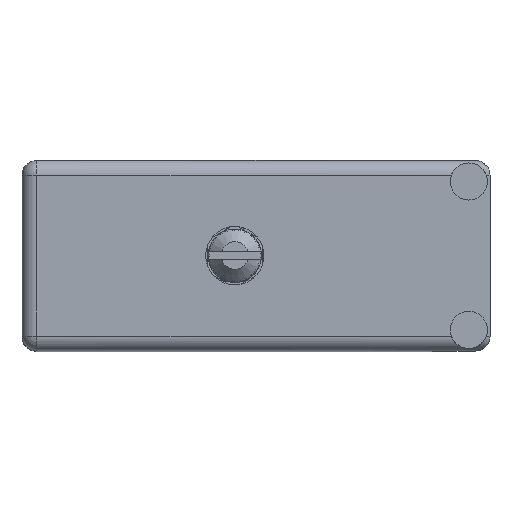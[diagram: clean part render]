
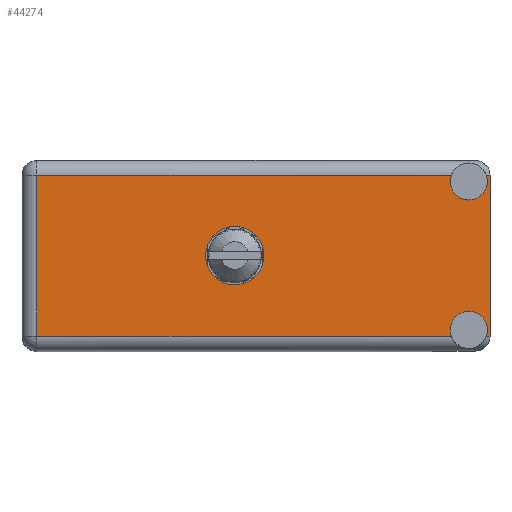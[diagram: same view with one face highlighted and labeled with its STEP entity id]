
A CAD part, top view. The second image highlights one B-rep face of the part: STEP entity #44274.
In plain terms, the highlighted face is planar.
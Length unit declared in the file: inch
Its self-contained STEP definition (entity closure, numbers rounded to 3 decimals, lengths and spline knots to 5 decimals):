
#1597 = AXIS2_PLACEMENT_3D ( 'NONE', #51165, #58360, #12794 ) ;
#5185 = DIRECTION ( 'NONE',  ( 1., 0., 0. ) ) ;
#5700 = EDGE_CURVE ( 'NONE', #101585, #38533, #28578, .T. ) ;
#5753 = DIRECTION ( 'NONE',  ( 0., 0., 1. ) ) ;
#6782 = ORIENTED_EDGE ( 'NONE', *, *, #45002, .F. ) ;
#7021 = EDGE_CURVE ( 'NONE', #78880, #65036, #67676, .T. ) ;
#10371 = CARTESIAN_POINT ( 'NONE',  ( 1.104, 1.466, -0.35 ) ) ;
#12250 = EDGE_CURVE ( 'NONE', #49900, #14841, #100233, .T. ) ;
#12794 = DIRECTION ( 'NONE',  ( 0., 0., 1. ) ) ;
#14841 = VERTEX_POINT ( 'NONE', #49491 ) ;
#14918 = EDGE_CURVE ( 'NONE', #27132, #76362, #71881, .T. ) ;
#15191 = CIRCLE ( 'NONE', #55643, 0.0875 ) ;
#15607 = LINE ( 'NONE', #66456, #87981 ) ;
#15711 = ORIENTED_EDGE ( 'NONE', *, *, #14918, .F. ) ;
#15985 = VERTEX_POINT ( 'NONE', #34496 ) ;
#16277 = VECTOR ( 'NONE', #5185, 39.37008 ) ;
#17382 = VECTOR ( 'NONE', #42668, 39.37008 ) ;
#18248 = CIRCLE ( 'NONE', #67312, 0.0875 ) ;
#18289 = DIRECTION ( 'NONE',  ( 0., 1., 0. ) ) ;
#20868 = ORIENTED_EDGE ( 'NONE', *, *, #64016, .F. ) ;
#20894 = DIRECTION ( 'NONE',  ( 0., 1., 0. ) ) ;
#21008 = DIRECTION ( 'NONE',  ( 0., 0., 1. ) ) ;
#21686 = EDGE_LOOP ( 'NONE', ( #95772, #64790 ) ) ;
#21742 = ORIENTED_EDGE ( 'NONE', *, *, #69128, .T. ) ;
#21962 = VECTOR ( 'NONE', #62475, 39.37008 ) ;
#23412 = LINE ( 'NONE', #81216, #17382 ) ;
#25297 = ORIENTED_EDGE ( 'NONE', *, *, #73729, .F. ) ;
#27132 = VERTEX_POINT ( 'NONE', #87765 ) ;
#28578 = LINE ( 'NONE', #98809, #16277 ) ;
#28747 = CARTESIAN_POINT ( 'NONE',  ( 0., 1.466, 0. ) ) ;
#29049 = DIRECTION ( 'NONE',  ( 0., 0., 1. ) ) ;
#29770 = FACE_BOUND ( 'NONE', #21686, .T. ) ;
#30309 = CARTESIAN_POINT ( 'NONE',  ( 1.204, 1.466, 0.3795 ) ) ;
#30442 = CARTESIAN_POINT ( 'NONE',  ( 1.104, 1.466, 0.35 ) ) ;
#30597 = CARTESIAN_POINT ( 'NONE',  ( -0.934, 1.466, -0.3795 ) ) ;
#31629 = CARTESIAN_POINT ( 'NONE',  ( -1.004, 1.466, -0.3795 ) ) ;
#34237 = EDGE_CURVE ( 'NONE', #14841, #49900, #58819, .T. ) ;
#34496 = CARTESIAN_POINT ( 'NONE',  ( 1.204, 1.466, -0.3795 ) ) ;
#34501 = LINE ( 'NONE', #52857, #44314 ) ;
#35379 = DIRECTION ( 'NONE',  ( -1., 0., 0. ) ) ;
#36099 = CARTESIAN_POINT ( 'NONE',  ( -1.004, 1.466, -0.3795 ) ) ;
#36655 = CARTESIAN_POINT ( 'NONE',  ( 1.02162, 1.466, -0.3795 ) ) ;
#38533 = VERTEX_POINT ( 'NONE', #99086 ) ;
#41197 = PLANE ( 'NONE',  #95051 ) ;
#42668 = DIRECTION ( 'NONE',  ( 1., 0., 0. ) ) ;
#42718 = LINE ( 'NONE', #31629, #21962 ) ;
#42878 = DIRECTION ( 'NONE',  ( 0., 1., 0. ) ) ;
#42951 = VECTOR ( 'NONE', #51216, 39.37008 ) ;
#43680 = VERTEX_POINT ( 'NONE', #87415 ) ;
#44274 = ADVANCED_FACE ( 'NONE', ( #29770, #66619 ), #41197, .T. ) ;
#44314 = VECTOR ( 'NONE', #21008, 39.37008 ) ;
#44689 = DIRECTION ( 'NONE',  ( 0., 0., 1. ) ) ;
#45002 = EDGE_CURVE ( 'NONE', #76362, #38533, #56584, .T. ) ;
#45811 = DIRECTION ( 'NONE',  ( 0., 1., 0. ) ) ;
#49491 = CARTESIAN_POINT ( 'NONE',  ( 0., 1.466, 0.1375 ) ) ;
#49900 = VERTEX_POINT ( 'NONE', #99537 ) ;
#50642 = EDGE_CURVE ( 'NONE', #27132, #92235, #23412, .T. ) ;
#51165 = CARTESIAN_POINT ( 'NONE',  ( 1.104, 1.466, 0.35 ) ) ;
#51216 = DIRECTION ( 'NONE',  ( -1., 0., 0. ) ) ;
#52857 = CARTESIAN_POINT ( 'NONE',  ( -0.934, 1.466, -0.4495 ) ) ;
#55420 = EDGE_CURVE ( 'NONE', #15985, #92235, #15607, .T. ) ;
#55643 = AXIS2_PLACEMENT_3D ( 'NONE', #60924, #69491, #29049 ) ;
#56584 = CIRCLE ( 'NONE', #60989, 0.0875 ) ;
#56597 = AXIS2_PLACEMENT_3D ( 'NONE', #68106, #69105, #44689 ) ;
#57465 = DIRECTION ( 'NONE',  ( 0., 0., 1. ) ) ;
#58360 = DIRECTION ( 'NONE',  ( 0., 1., 0. ) ) ;
#58819 = CIRCLE ( 'NONE', #56597, 0.1375 ) ;
#60924 = CARTESIAN_POINT ( 'NONE',  ( 1.104, 1.466, -0.35 ) ) ;
#60966 = EDGE_CURVE ( 'NONE', #65036, #101585, #34501, .T. ) ;
#60989 = AXIS2_PLACEMENT_3D ( 'NONE', #30442, #45811, #61628 ) ;
#61628 = DIRECTION ( 'NONE',  ( 0., 0., 1. ) ) ;
#62475 = DIRECTION ( 'NONE',  ( -1., 0., 0. ) ) ;
#62893 = ORIENTED_EDGE ( 'NONE', *, *, #50642, .T. ) ;
#63100 = AXIS2_PLACEMENT_3D ( 'NONE', #28747, #20894, #5753 ) ;
#64016 = EDGE_CURVE ( 'NONE', #78880, #43680, #18248, .T. ) ;
#64790 = ORIENTED_EDGE ( 'NONE', *, *, #12250, .F. ) ;
#65036 = VERTEX_POINT ( 'NONE', #30597 ) ;
#66456 = CARTESIAN_POINT ( 'NONE',  ( 1.204, 1.466, 0.4495 ) ) ;
#66492 = EDGE_LOOP ( 'NONE', ( #87865, #6782, #15711, #62893, #67953, #21742, #25297, #20868, #68590, #70917 ) ) ;
#66619 = FACE_OUTER_BOUND ( 'NONE', #66492, .T. ) ;
#67312 = AXIS2_PLACEMENT_3D ( 'NONE', #10371, #18289, #88842 ) ;
#67545 = CARTESIAN_POINT ( 'NONE',  ( 1.18638, 1.466, -0.3795 ) ) ;
#67676 = LINE ( 'NONE', #36099, #42951 ) ;
#67953 = ORIENTED_EDGE ( 'NONE', *, *, #55420, .F. ) ;
#68106 = CARTESIAN_POINT ( 'NONE',  ( 0., 1.466, 0. ) ) ;
#68590 = ORIENTED_EDGE ( 'NONE', *, *, #7021, .T. ) ;
#69105 = DIRECTION ( 'NONE',  ( 0., 1., 0. ) ) ;
#69128 = EDGE_CURVE ( 'NONE', #15985, #97114, #42718, .T. ) ;
#69491 = DIRECTION ( 'NONE',  ( 0., 1., 0. ) ) ;
#70917 = ORIENTED_EDGE ( 'NONE', *, *, #60966, .T. ) ;
#71881 = CIRCLE ( 'NONE', #1597, 0.0875 ) ;
#73729 = EDGE_CURVE ( 'NONE', #43680, #97114, #15191, .T. ) ;
#75691 = CARTESIAN_POINT ( 'NONE',  ( 1.104, 1.466, 0.2625 ) ) ;
#76362 = VERTEX_POINT ( 'NONE', #75691 ) ;
#78880 = VERTEX_POINT ( 'NONE', #36655 ) ;
#80922 = CARTESIAN_POINT ( 'NONE',  ( -0.934, 1.466, 0.3795 ) ) ;
#81216 = CARTESIAN_POINT ( 'NONE',  ( 1.204, 1.466, 0.3795 ) ) ;
#87415 = CARTESIAN_POINT ( 'NONE',  ( 1.104, 1.466, -0.2625 ) ) ;
#87765 = CARTESIAN_POINT ( 'NONE',  ( 1.18638, 1.466, 0.3795 ) ) ;
#87865 = ORIENTED_EDGE ( 'NONE', *, *, #5700, .T. ) ;
#87981 = VECTOR ( 'NONE', #57465, 39.37008 ) ;
#88842 = DIRECTION ( 'NONE',  ( 0., 0., 1. ) ) ;
#90955 = CARTESIAN_POINT ( 'NONE',  ( -1.004, 1.466, -0.4495 ) ) ;
#92235 = VERTEX_POINT ( 'NONE', #30309 ) ;
#95051 = AXIS2_PLACEMENT_3D ( 'NONE', #90955, #42878, #35379 ) ;
#95772 = ORIENTED_EDGE ( 'NONE', *, *, #34237, .F. ) ;
#97114 = VERTEX_POINT ( 'NONE', #67545 ) ;
#98809 = CARTESIAN_POINT ( 'NONE',  ( 1.204, 1.466, 0.3795 ) ) ;
#99086 = CARTESIAN_POINT ( 'NONE',  ( 1.02162, 1.466, 0.3795 ) ) ;
#99537 = CARTESIAN_POINT ( 'NONE',  ( 0., 1.466, -0.1375 ) ) ;
#100233 = CIRCLE ( 'NONE', #63100, 0.1375 ) ;
#101585 = VERTEX_POINT ( 'NONE', #80922 ) ;
